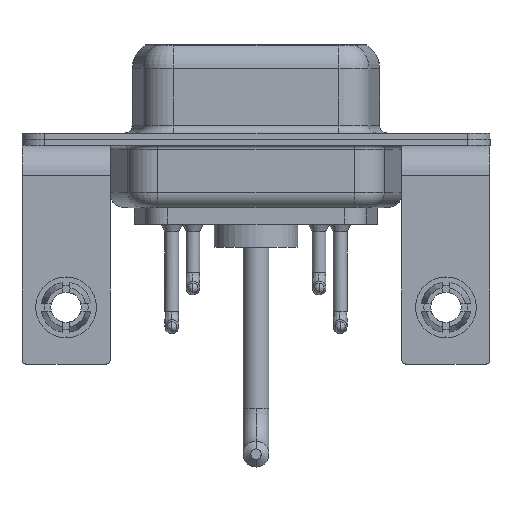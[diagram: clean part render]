
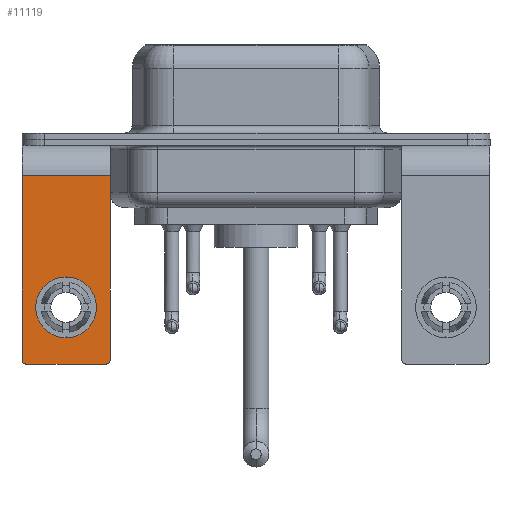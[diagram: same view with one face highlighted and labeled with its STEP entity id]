
A CAD part, front view. The second image highlights one B-rep face of the part: STEP entity #11119.
In plain terms, the highlighted planar face has unit normal (0, -1, 0).
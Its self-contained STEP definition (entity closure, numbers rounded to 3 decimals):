
#105 = CARTESIAN_POINT ( 'NONE',  ( 0., -6.25, -13.07 ) ) ;
#895 = CARTESIAN_POINT ( 'NONE',  ( 2.65, -6.25, -14.55 ) ) ;
#944 = DIRECTION ( 'NONE',  ( 0., 0., 1. ) ) ;
#1197 = ORIENTED_EDGE ( 'NONE', *, *, #10999, .T. ) ;
#1201 = AXIS2_PLACEMENT_3D ( 'NONE', #1247, #11382, #11478 ) ;
#1247 = CARTESIAN_POINT ( 'NONE',  ( 0., -6.25, -11.07 ) ) ;
#1278 = DIRECTION ( 'NONE',  ( 0., 0., -1. ) ) ;
#1636 = EDGE_CURVE ( 'NONE', #4328, #3160, #2712, .T. ) ;
#1778 = ORIENTED_EDGE ( 'NONE', *, *, #3926, .F. ) ;
#2178 = CIRCLE ( 'NONE', #17272, 2. ) ;
#2179 = DIRECTION ( 'NONE',  ( -1., 0., 0. ) ) ;
#2269 = CARTESIAN_POINT ( 'NONE',  ( -2.9, -6.25, -14.55 ) ) ;
#2411 = CIRCLE ( 'NONE', #6339, 0.25 ) ;
#2586 = ORIENTED_EDGE ( 'NONE', *, *, #1636, .T. ) ;
#2712 = LINE ( 'NONE', #18490, #9142 ) ;
#2852 = CARTESIAN_POINT ( 'NONE',  ( -2.9, -6.25, -2.4 ) ) ;
#3160 = VERTEX_POINT ( 'NONE', #2269 ) ;
#3617 = EDGE_CURVE ( 'NONE', #5439, #8752, #2411, .T. ) ;
#3681 = CARTESIAN_POINT ( 'NONE',  ( -2.65, -6.25, -14.8 ) ) ;
#3733 = CIRCLE ( 'NONE', #13992, 0.25 ) ;
#3889 = FACE_OUTER_BOUND ( 'NONE', #10225, .T. ) ;
#3926 = EDGE_CURVE ( 'NONE', #5439, #13423, #5998, .T. ) ;
#4062 = DIRECTION ( 'NONE',  ( 0., 0., -1. ) ) ;
#4328 = VERTEX_POINT ( 'NONE', #2852 ) ;
#4355 = ORIENTED_EDGE ( 'NONE', *, *, #3617, .T. ) ;
#4550 = CIRCLE ( 'NONE', #1201, 2. ) ;
#4556 = EDGE_CURVE ( 'NONE', #18317, #4328, #9565, .T. ) ;
#4645 = EDGE_CURVE ( 'NONE', #18317, #8752, #8246, .T. ) ;
#5086 = VECTOR ( 'NONE', #2179, 1000. ) ;
#5121 = FACE_BOUND ( 'NONE', #13086, .T. ) ;
#5210 = PLANE ( 'NONE',  #16399 ) ;
#5439 = VERTEX_POINT ( 'NONE', #16127 ) ;
#5918 = DIRECTION ( 'NONE',  ( 0., 0., 1. ) ) ;
#5998 = LINE ( 'NONE', #7319, #18409 ) ;
#6049 = EDGE_CURVE ( 'NONE', #8257, #6759, #2178, .T. ) ;
#6339 = AXIS2_PLACEMENT_3D ( 'NONE', #895, #6677, #7907 ) ;
#6387 = EDGE_CURVE ( 'NONE', #6759, #8257, #4550, .T. ) ;
#6677 = DIRECTION ( 'NONE',  ( 0., -1., 0. ) ) ;
#6759 = VERTEX_POINT ( 'NONE', #9768 ) ;
#7319 = CARTESIAN_POINT ( 'NONE',  ( 2.9, -6.25, -14.8 ) ) ;
#7907 = DIRECTION ( 'NONE',  ( 0., 0., 1. ) ) ;
#7960 = DIRECTION ( 'NONE',  ( 0., 1., 0. ) ) ;
#8246 = LINE ( 'NONE', #18419, #9336 ) ;
#8257 = VERTEX_POINT ( 'NONE', #105 ) ;
#8334 = CARTESIAN_POINT ( 'NONE',  ( 2.9, -6.25, -2.4 ) ) ;
#8752 = VERTEX_POINT ( 'NONE', #8894 ) ;
#8894 = CARTESIAN_POINT ( 'NONE',  ( 2.9, -6.25, -14.55 ) ) ;
#8914 = CARTESIAN_POINT ( 'NONE',  ( -2.65, -6.25, -14.55 ) ) ;
#9142 = VECTOR ( 'NONE', #1278, 1000. ) ;
#9336 = VECTOR ( 'NONE', #4062, 1000. ) ;
#9565 = LINE ( 'NONE', #12302, #5086 ) ;
#9768 = CARTESIAN_POINT ( 'NONE',  ( 0., -6.25, -9.07 ) ) ;
#10225 = EDGE_LOOP ( 'NONE', ( #2586, #1197, #1778, #4355, #14370, #14004 ) ) ;
#10417 = DIRECTION ( 'NONE',  ( 0., 0., 1. ) ) ;
#10458 = CARTESIAN_POINT ( 'NONE',  ( 0., -6.25, -11.07 ) ) ;
#10617 = DIRECTION ( 'NONE',  ( 0., -1., 0. ) ) ;
#10999 = EDGE_CURVE ( 'NONE', #3160, #13423, #3733, .T. ) ;
#11060 = ORIENTED_EDGE ( 'NONE', *, *, #6049, .T. ) ;
#11119 = ADVANCED_FACE ( 'NONE', ( #5121, #3889 ), #5210, .F. ) ;
#11382 = DIRECTION ( 'NONE',  ( 0., 1., 0. ) ) ;
#11478 = DIRECTION ( 'NONE',  ( 0., 0., 1. ) ) ;
#12302 = CARTESIAN_POINT ( 'NONE',  ( 2.9, -6.25, -2.4 ) ) ;
#12575 = ORIENTED_EDGE ( 'NONE', *, *, #6387, .T. ) ;
#13086 = EDGE_LOOP ( 'NONE', ( #11060, #12575 ) ) ;
#13423 = VERTEX_POINT ( 'NONE', #3681 ) ;
#13992 = AXIS2_PLACEMENT_3D ( 'NONE', #8914, #10617, #10417 ) ;
#14004 = ORIENTED_EDGE ( 'NONE', *, *, #4556, .T. ) ;
#14370 = ORIENTED_EDGE ( 'NONE', *, *, #4645, .F. ) ;
#15128 = CARTESIAN_POINT ( 'NONE',  ( 2.9, -6.25, -2.4 ) ) ;
#16127 = CARTESIAN_POINT ( 'NONE',  ( 2.65, -6.25, -14.8 ) ) ;
#16215 = DIRECTION ( 'NONE',  ( 0., 1., 0. ) ) ;
#16399 = AXIS2_PLACEMENT_3D ( 'NONE', #8334, #7960, #944 ) ;
#17272 = AXIS2_PLACEMENT_3D ( 'NONE', #10458, #16215, #5918 ) ;
#17608 = DIRECTION ( 'NONE',  ( -1., 0., 0. ) ) ;
#18317 = VERTEX_POINT ( 'NONE', #15128 ) ;
#18409 = VECTOR ( 'NONE', #17608, 1000. ) ;
#18419 = CARTESIAN_POINT ( 'NONE',  ( 2.9, -6.25, -2.4 ) ) ;
#18490 = CARTESIAN_POINT ( 'NONE',  ( -2.9, -6.25, -2.4 ) ) ;
